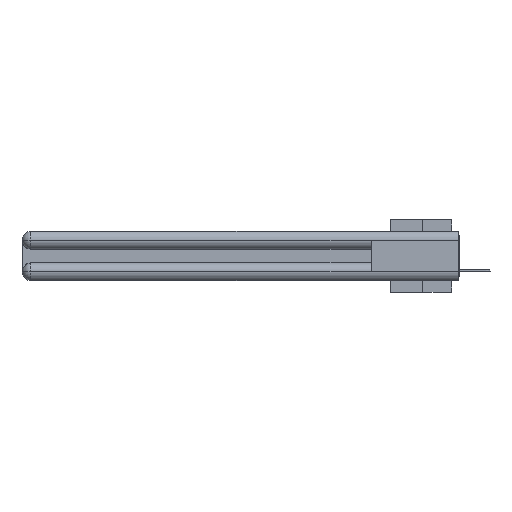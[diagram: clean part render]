
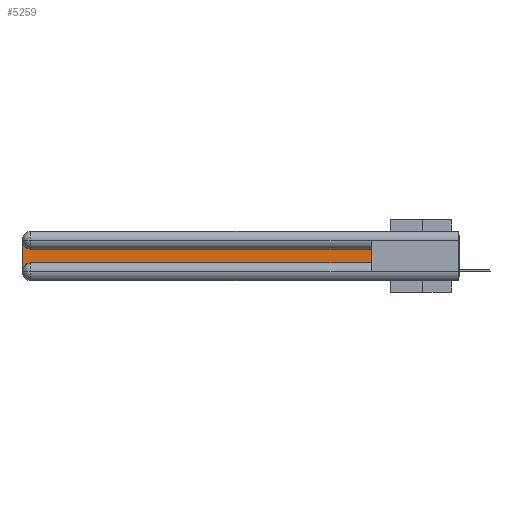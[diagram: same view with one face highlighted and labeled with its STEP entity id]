
A CAD part, left-side view. The second image highlights one B-rep face of the part: STEP entity #5259.
In plain terms, the highlighted planar face has unit normal (-1, 0, 0).
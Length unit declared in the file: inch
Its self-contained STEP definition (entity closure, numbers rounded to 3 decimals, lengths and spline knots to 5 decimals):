
#314 = VECTOR ( 'NONE', #27531, 39.37008 ) ;
#3064 = DIRECTION ( 'NONE',  ( 0., 0., -1. ) ) ;
#3237 = VECTOR ( 'NONE', #8321, 39.37008 ) ;
#3251 = CARTESIAN_POINT ( 'NONE',  ( 0.075, 2.94, -0.2175 ) ) ;
#5244 = EDGE_CURVE ( 'NONE', #37640, #38436, #8119, .T. ) ;
#5259 = ADVANCED_FACE ( 'NONE', ( #33579 ), #20935, .F. ) ;
#5329 = ORIENTED_EDGE ( 'NONE', *, *, #29591, .T. ) ;
#6602 = VECTOR ( 'NONE', #11033, 39.37008 ) ;
#6935 = CARTESIAN_POINT ( 'NONE',  ( 0.075, 0.6, -0.1225 ) ) ;
#7919 = CARTESIAN_POINT ( 'NONE',  ( 0.075, 3., -0.1225 ) ) ;
#8119 = LINE ( 'NONE', #29860, #3237 ) ;
#8139 = LINE ( 'NONE', #20750, #6602 ) ;
#8321 = DIRECTION ( 'NONE',  ( 0., 0., 1. ) ) ;
#8711 = VERTEX_POINT ( 'NONE', #3251 ) ;
#9097 = LINE ( 'NONE', #38268, #36479 ) ;
#11033 = DIRECTION ( 'NONE',  ( 0., 0., -1. ) ) ;
#11842 = VERTEX_POINT ( 'NONE', #21639 ) ;
#12665 = CARTESIAN_POINT ( 'NONE',  ( 0.075, 0.6, -0.2175 ) ) ;
#13760 = ORIENTED_EDGE ( 'NONE', *, *, #33565, .T. ) ;
#16551 = ORIENTED_EDGE ( 'NONE', *, *, #5244, .T. ) ;
#16807 = AXIS2_PLACEMENT_3D ( 'NONE', #31843, #38243, #3064 ) ;
#17592 = LINE ( 'NONE', #24015, #314 ) ;
#17629 = DIRECTION ( 'NONE',  ( 1., 0., 0. ) ) ;
#18621 = DIRECTION ( 'NONE',  ( 0., 1., 0. ) ) ;
#19097 = AXIS2_PLACEMENT_3D ( 'NONE', #7919, #17629, #30269 ) ;
#19430 = DIRECTION ( 'NONE',  ( 1., 0., 0. ) ) ;
#19752 = CARTESIAN_POINT ( 'NONE',  ( 0.075, 3., -0.2775 ) ) ;
#20315 = EDGE_CURVE ( 'NONE', #8711, #37640, #17592, .T. ) ;
#20750 = CARTESIAN_POINT ( 'NONE',  ( 0.075, 3., -0.2175 ) ) ;
#20935 = PLANE ( 'NONE',  #19097 ) ;
#21432 = CARTESIAN_POINT ( 'NONE',  ( 0.075, 2.94, -0.1225 ) ) ;
#21639 = CARTESIAN_POINT ( 'NONE',  ( 0.075, 3., -0.0625 ) ) ;
#21728 = EDGE_CURVE ( 'NONE', #27882, #11842, #32033, .T. ) ;
#23858 = ORIENTED_EDGE ( 'NONE', *, *, #21728, .T. ) ;
#24015 = CARTESIAN_POINT ( 'NONE',  ( 0.075, 0.6, -0.2175 ) ) ;
#24844 = DIRECTION ( 'NONE',  ( 0., 0., -1. ) ) ;
#27531 = DIRECTION ( 'NONE',  ( 0., -1., 0. ) ) ;
#27882 = VERTEX_POINT ( 'NONE', #21432 ) ;
#28001 = EDGE_CURVE ( 'NONE', #11842, #32201, #8139, .T. ) ;
#28363 = ORIENTED_EDGE ( 'NONE', *, *, #28001, .T. ) ;
#29591 = EDGE_CURVE ( 'NONE', #38436, #27882, #9097, .T. ) ;
#29860 = CARTESIAN_POINT ( 'NONE',  ( 0.075, 0.6, -0.2175 ) ) ;
#30269 = DIRECTION ( 'NONE',  ( 0., 0., -1. ) ) ;
#30709 = EDGE_LOOP ( 'NONE', ( #5329, #23858, #28363, #13760, #37225, #16551 ) ) ;
#31843 = CARTESIAN_POINT ( 'NONE',  ( 0.075, 2.94, -0.2775 ) ) ;
#32033 = CIRCLE ( 'NONE', #37321, 0.06 ) ;
#32201 = VERTEX_POINT ( 'NONE', #19752 ) ;
#33565 = EDGE_CURVE ( 'NONE', #32201, #8711, #39934, .T. ) ;
#33579 = FACE_OUTER_BOUND ( 'NONE', #30709, .T. ) ;
#36479 = VECTOR ( 'NONE', #18621, 39.37008 ) ;
#37225 = ORIENTED_EDGE ( 'NONE', *, *, #20315, .T. ) ;
#37321 = AXIS2_PLACEMENT_3D ( 'NONE', #40547, #19430, #24844 ) ;
#37640 = VERTEX_POINT ( 'NONE', #12665 ) ;
#38243 = DIRECTION ( 'NONE',  ( 1., 0., 0. ) ) ;
#38268 = CARTESIAN_POINT ( 'NONE',  ( 0.075, 0.6, -0.1225 ) ) ;
#38436 = VERTEX_POINT ( 'NONE', #6935 ) ;
#39934 = CIRCLE ( 'NONE', #16807, 0.06 ) ;
#40547 = CARTESIAN_POINT ( 'NONE',  ( 0.075, 2.94, -0.0625 ) ) ;
